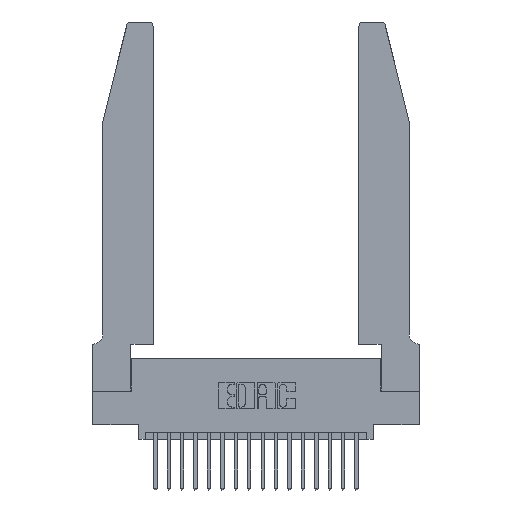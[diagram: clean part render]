
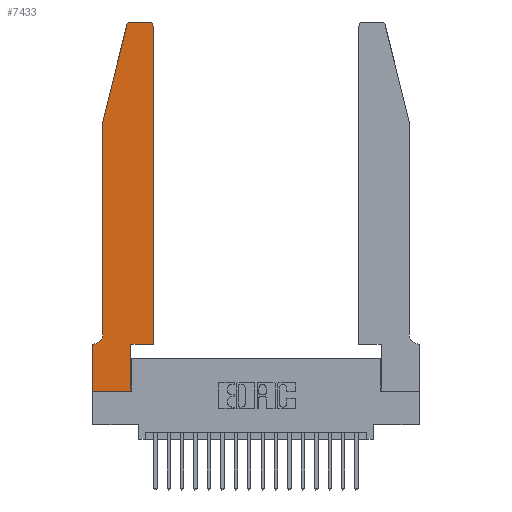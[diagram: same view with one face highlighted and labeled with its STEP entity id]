
A CAD part, top view. The second image highlights one B-rep face of the part: STEP entity #7433.
In plain terms, the highlighted planar face has unit normal (0, 0, 1).
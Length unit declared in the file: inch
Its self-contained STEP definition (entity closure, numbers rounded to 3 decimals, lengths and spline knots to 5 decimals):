
#25 = CARTESIAN_POINT ( 'NONE',  ( 0.0055, 0.42, 0.37 ) ) ;
#333 = ORIENTED_EDGE ( 'NONE', *, *, #4510, .T. ) ;
#389 = CARTESIAN_POINT ( 'NONE',  ( 0.4505, 0.35, 0.37 ) ) ;
#390 = VERTEX_POINT ( 'NONE', #13239 ) ;
#902 = DIRECTION ( 'NONE',  ( 1., 0., 0. ) ) ;
#993 = ORIENTED_EDGE ( 'NONE', *, *, #6459, .T. ) ;
#1240 = ORIENTED_EDGE ( 'NONE', *, *, #16466, .T. ) ;
#1401 = CARTESIAN_POINT ( 'NONE',  ( 0.4505, 0.35, 0.37 ) ) ;
#1733 = DIRECTION ( 'NONE',  ( -1., 0., 0. ) ) ;
#2169 = VECTOR ( 'NONE', #18584, 39.37008 ) ;
#2393 = ORIENTED_EDGE ( 'NONE', *, *, #8052, .T. ) ;
#3131 = ORIENTED_EDGE ( 'NONE', *, *, #16415, .T. ) ;
#3135 = CARTESIAN_POINT ( 'NONE',  ( 0.0755, 0.35, 0.37 ) ) ;
#3312 = DIRECTION ( 'NONE',  ( 0., 0., 1. ) ) ;
#3401 = VERTEX_POINT ( 'NONE', #13237 ) ;
#3547 = ORIENTED_EDGE ( 'NONE', *, *, #4905, .T. ) ;
#3618 = VERTEX_POINT ( 'NONE', #17675 ) ;
#3739 = ORIENTED_EDGE ( 'NONE', *, *, #4246, .T. ) ;
#3908 = CARTESIAN_POINT ( 'NONE',  ( 0.4505, 0.35, 0.37 ) ) ;
#4163 = CARTESIAN_POINT ( 'NONE',  ( 0.2605, 2.75, 0.37 ) ) ;
#4246 = EDGE_CURVE ( 'NONE', #3401, #15949, #13858, .T. ) ;
#4281 = ORIENTED_EDGE ( 'NONE', *, *, #16564, .T. ) ;
#4510 = EDGE_CURVE ( 'NONE', #3618, #17971, #13615, .T. ) ;
#4757 = CARTESIAN_POINT ( 'NONE',  ( 0.4205, 2.75, 0.37 ) ) ;
#4905 = EDGE_CURVE ( 'NONE', #390, #3618, #18880, .T. ) ;
#5180 = EDGE_LOOP ( 'NONE', ( #4281, #10760, #3131, #1240, #9514, #3739, #16823, #2393, #3547, #333, #11905, #993 ) ) ;
#5421 = CARTESIAN_POINT ( 'NONE',  ( 0.0755, 2., 0.37 ) ) ;
#5552 = DIRECTION ( 'NONE',  ( 0., -1., 0. ) ) ;
#5677 = AXIS2_PLACEMENT_3D ( 'NONE', #9075, #20307, #10674 ) ;
#6133 = VERTEX_POINT ( 'NONE', #4757 ) ;
#6135 = VECTOR ( 'NONE', #9908, 39.37008 ) ;
#6385 = CARTESIAN_POINT ( 'NONE',  ( 0.2865, 0.35, 0.37 ) ) ;
#6459 = EDGE_CURVE ( 'NONE', #17263, #6133, #7275, .T. ) ;
#6803 = CARTESIAN_POINT ( 'NONE',  ( 0.284, 2.75, 0.37 ) ) ;
#7275 = CIRCLE ( 'NONE', #12205, 0.03 ) ;
#7433 = ADVANCED_FACE ( 'NONE', ( #14748 ), #9705, .T. ) ;
#8052 = EDGE_CURVE ( 'NONE', #9339, #390, #20744, .T. ) ;
#8172 = CARTESIAN_POINT ( 'NONE',  ( 0., 0., 0.37 ) ) ;
#8633 = DIRECTION ( 'NONE',  ( 1., 0., 0. ) ) ;
#8935 = CIRCLE ( 'NONE', #10502, 0.07 ) ;
#9075 = CARTESIAN_POINT ( 'NONE',  ( 0.284, 2.72, 0.37 ) ) ;
#9339 = VERTEX_POINT ( 'NONE', #13164 ) ;
#9514 = ORIENTED_EDGE ( 'NONE', *, *, #19214, .T. ) ;
#9597 = VECTOR ( 'NONE', #9607, 39.37008 ) ;
#9607 = DIRECTION ( 'NONE',  ( -1., 0., 0. ) ) ;
#9705 = PLANE ( 'NONE',  #9936 ) ;
#9768 = LINE ( 'NONE', #3908, #2169 ) ;
#9908 = DIRECTION ( 'NONE',  ( 0., -1., 0. ) ) ;
#9936 = AXIS2_PLACEMENT_3D ( 'NONE', #14481, #3312, #14557 ) ;
#10051 = VECTOR ( 'NONE', #19900, 39.37008 ) ;
#10502 = AXIS2_PLACEMENT_3D ( 'NONE', #25, #11427, #1733 ) ;
#10647 = DIRECTION ( 'NONE',  ( 0., 0., 1. ) ) ;
#10674 = DIRECTION ( 'NONE',  ( 1., 0., 0. ) ) ;
#10760 = ORIENTED_EDGE ( 'NONE', *, *, #20237, .T. ) ;
#11427 = DIRECTION ( 'NONE',  ( 0., 0., -1. ) ) ;
#11809 = VECTOR ( 'NONE', #17050, 39.37008 ) ;
#11905 = ORIENTED_EDGE ( 'NONE', *, *, #16045, .T. ) ;
#12205 = AXIS2_PLACEMENT_3D ( 'NONE', #20276, #10647, #902 ) ;
#13164 = CARTESIAN_POINT ( 'NONE',  ( 0., 0., 0.37 ) ) ;
#13178 = EDGE_CURVE ( 'NONE', #15949, #9339, #14682, .T. ) ;
#13237 = CARTESIAN_POINT ( 'NONE',  ( 0.0055, 0.35, 0.37 ) ) ;
#13239 = CARTESIAN_POINT ( 'NONE',  ( 0.2865, 0., 0.37 ) ) ;
#13615 = LINE ( 'NONE', #389, #17410 ) ;
#13847 = CARTESIAN_POINT ( 'NONE',  ( 0.0755, 0.42, 0.37 ) ) ;
#13858 = LINE ( 'NONE', #3135, #9597 ) ;
#14258 = CARTESIAN_POINT ( 'NONE',  ( 0.0755, 2., 0.37 ) ) ;
#14327 = LINE ( 'NONE', #5421, #10051 ) ;
#14389 = CARTESIAN_POINT ( 'NONE',  ( 0., 0., 0.37 ) ) ;
#14481 = CARTESIAN_POINT ( 'NONE',  ( 0., 0.35, 0.37 ) ) ;
#14548 = VERTEX_POINT ( 'NONE', #13847 ) ;
#14557 = DIRECTION ( 'NONE',  ( 1., 0., 0. ) ) ;
#14682 = LINE ( 'NONE', #8172, #6135 ) ;
#14748 = FACE_OUTER_BOUND ( 'NONE', #5180, .T. ) ;
#15585 = CARTESIAN_POINT ( 'NONE',  ( 0.4505, 2.72, 0.37 ) ) ;
#15949 = VERTEX_POINT ( 'NONE', #19779 ) ;
#15950 = CIRCLE ( 'NONE', #5677, 0.03 ) ;
#16033 = DIRECTION ( 'NONE',  ( 1., 0., 0. ) ) ;
#16045 = EDGE_CURVE ( 'NONE', #17971, #17263, #9768, .T. ) ;
#16115 = LINE ( 'NONE', #4163, #11809 ) ;
#16415 = EDGE_CURVE ( 'NONE', #19898, #20532, #14327, .T. ) ;
#16466 = EDGE_CURVE ( 'NONE', #20532, #14548, #17628, .T. ) ;
#16564 = EDGE_CURVE ( 'NONE', #6133, #18151, #16115, .T. ) ;
#16823 = ORIENTED_EDGE ( 'NONE', *, *, #13178, .T. ) ;
#17050 = DIRECTION ( 'NONE',  ( -1., 0., 0. ) ) ;
#17263 = VERTEX_POINT ( 'NONE', #15585 ) ;
#17410 = VECTOR ( 'NONE', #8633, 39.37008 ) ;
#17628 = LINE ( 'NONE', #18364, #18132 ) ;
#17675 = CARTESIAN_POINT ( 'NONE',  ( 0.2865, 0.35, 0.37 ) ) ;
#17900 = VECTOR ( 'NONE', #20826, 39.37008 ) ;
#17908 = CARTESIAN_POINT ( 'NONE',  ( 0.25487, 2.72718, 0.37 ) ) ;
#17971 = VERTEX_POINT ( 'NONE', #1401 ) ;
#18132 = VECTOR ( 'NONE', #5552, 39.37008 ) ;
#18151 = VERTEX_POINT ( 'NONE', #6803 ) ;
#18364 = CARTESIAN_POINT ( 'NONE',  ( 0.0755, 2., 0.37 ) ) ;
#18584 = DIRECTION ( 'NONE',  ( 0., 1., 0. ) ) ;
#18880 = LINE ( 'NONE', #6385, #17900 ) ;
#19214 = EDGE_CURVE ( 'NONE', #14548, #3401, #8935, .T. ) ;
#19779 = CARTESIAN_POINT ( 'NONE',  ( 0., 0.35, 0.37 ) ) ;
#19898 = VERTEX_POINT ( 'NONE', #17908 ) ;
#19900 = DIRECTION ( 'NONE',  ( -0.239, -0.971, 0. ) ) ;
#20237 = EDGE_CURVE ( 'NONE', #18151, #19898, #15950, .T. ) ;
#20243 = VECTOR ( 'NONE', #16033, 39.37008 ) ;
#20276 = CARTESIAN_POINT ( 'NONE',  ( 0.4205, 2.72, 0.37 ) ) ;
#20307 = DIRECTION ( 'NONE',  ( 0., 0., 1. ) ) ;
#20532 = VERTEX_POINT ( 'NONE', #14258 ) ;
#20744 = LINE ( 'NONE', #14389, #20243 ) ;
#20826 = DIRECTION ( 'NONE',  ( 0., 1., 0. ) ) ;
